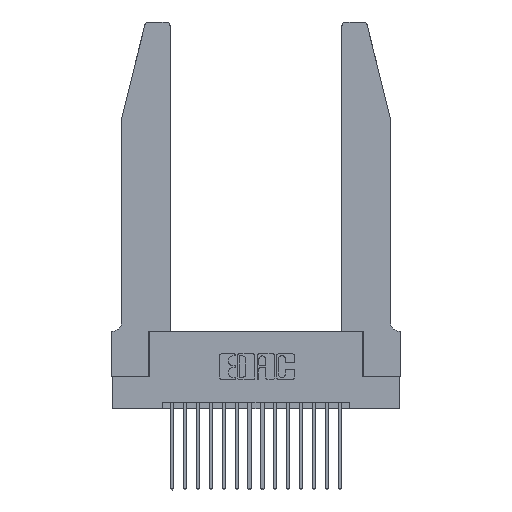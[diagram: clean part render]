
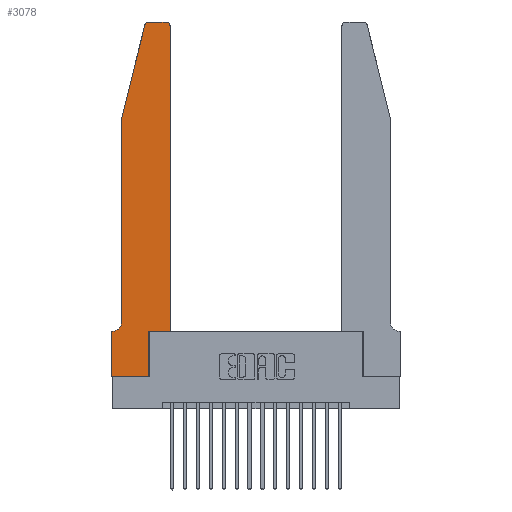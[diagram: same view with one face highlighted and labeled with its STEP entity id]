
A CAD part, top view. The second image highlights one B-rep face of the part: STEP entity #3078.
In plain terms, the highlighted planar face has unit normal (0, 0, 1).
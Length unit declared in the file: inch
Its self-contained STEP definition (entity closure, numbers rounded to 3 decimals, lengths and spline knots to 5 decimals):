
#99 = VECTOR ( 'NONE', #13550, 39.37008 ) ;
#151 = VECTOR ( 'NONE', #11215, 39.37008 ) ;
#436 = VERTEX_POINT ( 'NONE', #5852 ) ;
#594 = CARTESIAN_POINT ( 'NONE',  ( 0.2605, 2.75, 0.37 ) ) ;
#691 = VERTEX_POINT ( 'NONE', #5956 ) ;
#900 = EDGE_LOOP ( 'NONE', ( #7054, #1456, #7625, #18204, #2025, #18440, #17113, #4793, #7152, #13959, #10970, #12080 ) ) ;
#1065 = LINE ( 'NONE', #12026, #99 ) ;
#1145 = VERTEX_POINT ( 'NONE', #5660 ) ;
#1214 = VERTEX_POINT ( 'NONE', #13737 ) ;
#1456 = ORIENTED_EDGE ( 'NONE', *, *, #6000, .T. ) ;
#1564 = DIRECTION ( 'NONE',  ( 1., 0., 0. ) ) ;
#1633 = EDGE_CURVE ( 'NONE', #691, #9702, #2073, .T. ) ;
#1696 = DIRECTION ( 'NONE',  ( 0., 0., 1. ) ) ;
#1736 = LINE ( 'NONE', #594, #4318 ) ;
#1770 = DIRECTION ( 'NONE',  ( 0., 1., 0. ) ) ;
#1915 = DIRECTION ( 'NONE',  ( -1., 0., 0. ) ) ;
#2009 = DIRECTION ( 'NONE',  ( 0., 0., -1. ) ) ;
#2025 = ORIENTED_EDGE ( 'NONE', *, *, #9851, .T. ) ;
#2073 = LINE ( 'NONE', #2268, #151 ) ;
#2268 = CARTESIAN_POINT ( 'NONE',  ( 0.0755, 2., 0.37 ) ) ;
#2888 = LINE ( 'NONE', #19514, #14237 ) ;
#3078 = ADVANCED_FACE ( 'NONE', ( #8367 ), #9371, .T. ) ;
#3171 = EDGE_CURVE ( 'NONE', #1145, #19444, #5325, .T. ) ;
#3361 = CARTESIAN_POINT ( 'NONE',  ( 0.0055, 0.35, 0.37 ) ) ;
#3379 = DIRECTION ( 'NONE',  ( 0., 0., 1. ) ) ;
#3556 = CARTESIAN_POINT ( 'NONE',  ( 0., 0., 0.37 ) ) ;
#3964 = EDGE_CURVE ( 'NONE', #5741, #9550, #12620, .T. ) ;
#3966 = EDGE_CURVE ( 'NONE', #19444, #436, #1065, .T. ) ;
#4318 = VECTOR ( 'NONE', #11136, 39.37008 ) ;
#4793 = ORIENTED_EDGE ( 'NONE', *, *, #3171, .T. ) ;
#4903 = CARTESIAN_POINT ( 'NONE',  ( 0.0055, 0.42, 0.37 ) ) ;
#4978 = DIRECTION ( 'NONE',  ( 1., 0., 0. ) ) ;
#5150 = DIRECTION ( 'NONE',  ( 0., -1., 0. ) ) ;
#5325 = LINE ( 'NONE', #14449, #14285 ) ;
#5471 = VERTEX_POINT ( 'NONE', #6581 ) ;
#5660 = CARTESIAN_POINT ( 'NONE',  ( 0., 0., 0.37 ) ) ;
#5741 = VERTEX_POINT ( 'NONE', #11512 ) ;
#5775 = VECTOR ( 'NONE', #1915, 39.37008 ) ;
#5852 = CARTESIAN_POINT ( 'NONE',  ( 0.2865, 0.35, 0.37 ) ) ;
#5956 = CARTESIAN_POINT ( 'NONE',  ( 0.25487, 2.72718, 0.37 ) ) ;
#6000 = EDGE_CURVE ( 'NONE', #10245, #691, #12161, .T. ) ;
#6407 = DIRECTION ( 'NONE',  ( -1., 0., 0. ) ) ;
#6581 = CARTESIAN_POINT ( 'NONE',  ( 0., 0.35, 0.37 ) ) ;
#6698 = EDGE_CURVE ( 'NONE', #5471, #1145, #10260, .T. ) ;
#7054 = ORIENTED_EDGE ( 'NONE', *, *, #8363, .T. ) ;
#7107 = EDGE_CURVE ( 'NONE', #13964, #5471, #16655, .T. ) ;
#7152 = ORIENTED_EDGE ( 'NONE', *, *, #3966, .T. ) ;
#7275 = CARTESIAN_POINT ( 'NONE',  ( 0.4505, 2.72, 0.37 ) ) ;
#7486 = CARTESIAN_POINT ( 'NONE',  ( 0., 0.35, 0.37 ) ) ;
#7625 = ORIENTED_EDGE ( 'NONE', *, *, #1633, .T. ) ;
#7642 = DIRECTION ( 'NONE',  ( 0., -1., 0. ) ) ;
#7803 = AXIS2_PLACEMENT_3D ( 'NONE', #7486, #1696, #1564 ) ;
#7860 = CARTESIAN_POINT ( 'NONE',  ( 0.4205, 2.72, 0.37 ) ) ;
#8363 = EDGE_CURVE ( 'NONE', #13806, #10245, #1736, .T. ) ;
#8367 = FACE_OUTER_BOUND ( 'NONE', #900, .T. ) ;
#8505 = DIRECTION ( 'NONE',  ( 1., 0., 0. ) ) ;
#8640 = EDGE_CURVE ( 'NONE', #436, #5741, #2888, .T. ) ;
#9341 = CARTESIAN_POINT ( 'NONE',  ( 0.2865, 0., 0.37 ) ) ;
#9371 = PLANE ( 'NONE',  #7803 ) ;
#9550 = VERTEX_POINT ( 'NONE', #7275 ) ;
#9702 = VERTEX_POINT ( 'NONE', #13716 ) ;
#9791 = EDGE_CURVE ( 'NONE', #9550, #13806, #12259, .T. ) ;
#9851 = EDGE_CURVE ( 'NONE', #1214, #13964, #19151, .T. ) ;
#10245 = VERTEX_POINT ( 'NONE', #11403 ) ;
#10260 = LINE ( 'NONE', #3556, #12859 ) ;
#10435 = VECTOR ( 'NONE', #7642, 39.37008 ) ;
#10970 = ORIENTED_EDGE ( 'NONE', *, *, #3964, .T. ) ;
#11136 = DIRECTION ( 'NONE',  ( -1., 0., 0. ) ) ;
#11143 = LINE ( 'NONE', #15281, #10435 ) ;
#11215 = DIRECTION ( 'NONE',  ( -0.239, -0.971, 0. ) ) ;
#11403 = CARTESIAN_POINT ( 'NONE',  ( 0.284, 2.75, 0.37 ) ) ;
#11512 = CARTESIAN_POINT ( 'NONE',  ( 0.4505, 0.35, 0.37 ) ) ;
#11662 = DIRECTION ( 'NONE',  ( 1., 0., 0. ) ) ;
#11742 = AXIS2_PLACEMENT_3D ( 'NONE', #7860, #3379, #15589 ) ;
#12026 = CARTESIAN_POINT ( 'NONE',  ( 0.2865, 0.35, 0.37 ) ) ;
#12030 = AXIS2_PLACEMENT_3D ( 'NONE', #15591, #12543, #4978 ) ;
#12080 = ORIENTED_EDGE ( 'NONE', *, *, #9791, .T. ) ;
#12161 = CIRCLE ( 'NONE', #12030, 0.03 ) ;
#12259 = CIRCLE ( 'NONE', #11742, 0.03 ) ;
#12543 = DIRECTION ( 'NONE',  ( 0., 0., 1. ) ) ;
#12620 = LINE ( 'NONE', #18258, #14511 ) ;
#12859 = VECTOR ( 'NONE', #5150, 39.37008 ) ;
#13550 = DIRECTION ( 'NONE',  ( 0., 1., 0. ) ) ;
#13716 = CARTESIAN_POINT ( 'NONE',  ( 0.0755, 2., 0.37 ) ) ;
#13737 = CARTESIAN_POINT ( 'NONE',  ( 0.0755, 0.42, 0.37 ) ) ;
#13806 = VERTEX_POINT ( 'NONE', #18215 ) ;
#13959 = ORIENTED_EDGE ( 'NONE', *, *, #8640, .T. ) ;
#13964 = VERTEX_POINT ( 'NONE', #3361 ) ;
#14237 = VECTOR ( 'NONE', #11662, 39.37008 ) ;
#14285 = VECTOR ( 'NONE', #8505, 39.37008 ) ;
#14449 = CARTESIAN_POINT ( 'NONE',  ( 0., 0., 0.37 ) ) ;
#14511 = VECTOR ( 'NONE', #1770, 39.37008 ) ;
#15281 = CARTESIAN_POINT ( 'NONE',  ( 0.0755, 2., 0.37 ) ) ;
#15589 = DIRECTION ( 'NONE',  ( 1., 0., 0. ) ) ;
#15591 = CARTESIAN_POINT ( 'NONE',  ( 0.284, 2.72, 0.37 ) ) ;
#16085 = AXIS2_PLACEMENT_3D ( 'NONE', #4903, #2009, #6407 ) ;
#16655 = LINE ( 'NONE', #18467, #5775 ) ;
#17113 = ORIENTED_EDGE ( 'NONE', *, *, #6698, .T. ) ;
#18204 = ORIENTED_EDGE ( 'NONE', *, *, #19299, .T. ) ;
#18215 = CARTESIAN_POINT ( 'NONE',  ( 0.4205, 2.75, 0.37 ) ) ;
#18258 = CARTESIAN_POINT ( 'NONE',  ( 0.4505, 0.35, 0.37 ) ) ;
#18440 = ORIENTED_EDGE ( 'NONE', *, *, #7107, .T. ) ;
#18467 = CARTESIAN_POINT ( 'NONE',  ( 0.0755, 0.35, 0.37 ) ) ;
#19151 = CIRCLE ( 'NONE', #16085, 0.07 ) ;
#19299 = EDGE_CURVE ( 'NONE', #9702, #1214, #11143, .T. ) ;
#19444 = VERTEX_POINT ( 'NONE', #9341 ) ;
#19514 = CARTESIAN_POINT ( 'NONE',  ( 0.4505, 0.35, 0.37 ) ) ;
